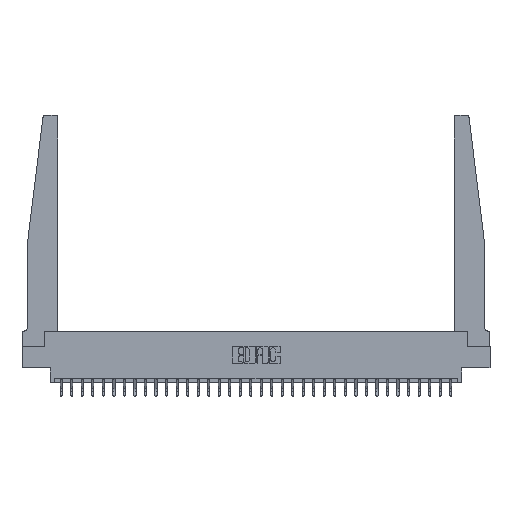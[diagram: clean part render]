
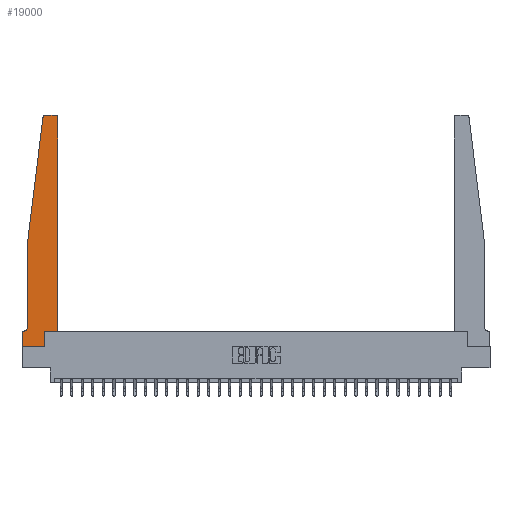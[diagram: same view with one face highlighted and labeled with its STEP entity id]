
A CAD part, top view. The second image highlights one B-rep face of the part: STEP entity #19000.
In plain terms, the highlighted planar face has unit normal (0, 0, 1).
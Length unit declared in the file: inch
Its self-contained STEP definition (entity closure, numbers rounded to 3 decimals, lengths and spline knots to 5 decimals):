
#228 = ORIENTED_EDGE ( 'NONE', *, *, #20052, .T. ) ;
#772 = CARTESIAN_POINT ( 'NONE',  ( 0.2605, 0.18, 0.37 ) ) ;
#920 = DIRECTION ( 'NONE',  ( 0., 1., 0. ) ) ;
#1320 = ORIENTED_EDGE ( 'NONE', *, *, #6253, .T. ) ;
#2026 = VECTOR ( 'NONE', #7015, 39.37008 ) ;
#2104 = AXIS2_PLACEMENT_3D ( 'NONE', #2556, #12099, #26341 ) ;
#2418 = VERTEX_POINT ( 'NONE', #26243 ) ;
#2556 = CARTESIAN_POINT ( 'NONE',  ( 0.015, 0.2375, 0.37 ) ) ;
#3016 = CARTESIAN_POINT ( 'NONE',  ( 0.425, 2.72, 0.37 ) ) ;
#3217 = LINE ( 'NONE', #29176, #16742 ) ;
#3379 = ORIENTED_EDGE ( 'NONE', *, *, #28128, .T. ) ;
#3583 = VERTEX_POINT ( 'NONE', #9162 ) ;
#3828 = DIRECTION ( 'NONE',  ( 1., 0., 0. ) ) ;
#4292 = VECTOR ( 'NONE', #920, 39.37008 ) ;
#4565 = CARTESIAN_POINT ( 'NONE',  ( 0.27653, 2.72, 0.37 ) ) ;
#4827 = EDGE_CURVE ( 'NONE', #3583, #15010, #14990, .T. ) ;
#4882 = DIRECTION ( 'NONE',  ( 1., 0., 0. ) ) ;
#4998 = CIRCLE ( 'NONE', #2104, 0.05 ) ;
#5313 = LINE ( 'NONE', #772, #13185 ) ;
#5626 = CARTESIAN_POINT ( 'NONE',  ( 0.425, 0.18, 0.37 ) ) ;
#5754 = DIRECTION ( 'NONE',  ( 0., 0., 1. ) ) ;
#5775 = CARTESIAN_POINT ( 'NONE',  ( 0.425, 0.18, 0.37 ) ) ;
#6186 = CARTESIAN_POINT ( 'NONE',  ( 0., 0.1875, 0.37 ) ) ;
#6253 = EDGE_CURVE ( 'NONE', #8029, #3583, #12339, .T. ) ;
#7015 = DIRECTION ( 'NONE',  ( 0., -1., 0. ) ) ;
#7041 = EDGE_CURVE ( 'NONE', #10366, #22657, #21961, .T. ) ;
#7259 = CIRCLE ( 'NONE', #21730, 0.03 ) ;
#7841 = CARTESIAN_POINT ( 'NONE',  ( 0.27653, 2.75, 0.37 ) ) ;
#8029 = VERTEX_POINT ( 'NONE', #20749 ) ;
#8044 = VERTEX_POINT ( 'NONE', #16354 ) ;
#8095 = LINE ( 'NONE', #12914, #13352 ) ;
#8832 = VERTEX_POINT ( 'NONE', #19907 ) ;
#9162 = CARTESIAN_POINT ( 'NONE',  ( 0.425, 0.18, 0.37 ) ) ;
#9662 = LINE ( 'NONE', #16986, #2026 ) ;
#9875 = ORIENTED_EDGE ( 'NONE', *, *, #13506, .T. ) ;
#10366 = VERTEX_POINT ( 'NONE', #27850 ) ;
#10538 = ORIENTED_EDGE ( 'NONE', *, *, #28315, .T. ) ;
#10979 = VECTOR ( 'NONE', #12352, 39.37008 ) ;
#11277 = VECTOR ( 'NONE', #29229, 39.37008 ) ;
#11292 = CIRCLE ( 'NONE', #11801, 0.03 ) ;
#11801 = AXIS2_PLACEMENT_3D ( 'NONE', #29205, #5754, #29053 ) ;
#11975 = ORIENTED_EDGE ( 'NONE', *, *, #13963, .T. ) ;
#12059 = VERTEX_POINT ( 'NONE', #25987 ) ;
#12060 = LINE ( 'NONE', #29104, #24418 ) ;
#12099 = DIRECTION ( 'NONE',  ( 0., 0., -1. ) ) ;
#12259 = EDGE_CURVE ( 'NONE', #12869, #8029, #5313, .T. ) ;
#12339 = LINE ( 'NONE', #5626, #11277 ) ;
#12352 = DIRECTION ( 'NONE',  ( -1., 0., 0. ) ) ;
#12611 = DIRECTION ( 'NONE',  ( 0., -1., 0. ) ) ;
#12739 = DIRECTION ( 'NONE',  ( -0.122, -0.992, 0. ) ) ;
#12869 = VERTEX_POINT ( 'NONE', #27484 ) ;
#12914 = CARTESIAN_POINT ( 'NONE',  ( 0.065, 1.25, 0.37 ) ) ;
#13185 = VECTOR ( 'NONE', #24089, 39.37008 ) ;
#13352 = VECTOR ( 'NONE', #12611, 39.37008 ) ;
#13506 = EDGE_CURVE ( 'NONE', #22657, #8832, #7259, .T. ) ;
#13808 = FACE_OUTER_BOUND ( 'NONE', #25601, .T. ) ;
#13877 = CARTESIAN_POINT ( 'NONE',  ( 0.015, 0.1875, 0.37 ) ) ;
#13963 = EDGE_CURVE ( 'NONE', #15010, #10366, #11292, .T. ) ;
#14781 = VECTOR ( 'NONE', #29008, 39.37008 ) ;
#14919 = CARTESIAN_POINT ( 'NONE',  ( 0.25, 2.75, 0.37 ) ) ;
#14990 = LINE ( 'NONE', #5775, #4292 ) ;
#15010 = VERTEX_POINT ( 'NONE', #3016 ) ;
#15713 = DIRECTION ( 'NONE',  ( 0., 0., 1. ) ) ;
#16354 = CARTESIAN_POINT ( 'NONE',  ( 0., 0., 0.37 ) ) ;
#16742 = VECTOR ( 'NONE', #12739, 39.37008 ) ;
#16812 = VERTEX_POINT ( 'NONE', #13877 ) ;
#16986 = CARTESIAN_POINT ( 'NONE',  ( 0., 0., 0.37 ) ) ;
#19000 = ADVANCED_FACE ( 'NONE', ( #13808 ), #27603, .T. ) ;
#19087 = DIRECTION ( 'NONE',  ( 0., 0., 1. ) ) ;
#19552 = VERTEX_POINT ( 'NONE', #25149 ) ;
#19609 = ORIENTED_EDGE ( 'NONE', *, *, #12259, .T. ) ;
#19646 = ORIENTED_EDGE ( 'NONE', *, *, #25704, .T. ) ;
#19907 = CARTESIAN_POINT ( 'NONE',  ( 0.24675, 2.72367, 0.37 ) ) ;
#20052 = EDGE_CURVE ( 'NONE', #8832, #2418, #3217, .T. ) ;
#20749 = CARTESIAN_POINT ( 'NONE',  ( 0.2605, 0.18, 0.37 ) ) ;
#21591 = CARTESIAN_POINT ( 'NONE',  ( 0.065, 0.1875, 0.37 ) ) ;
#21730 = AXIS2_PLACEMENT_3D ( 'NONE', #4565, #19087, #28182 ) ;
#21961 = LINE ( 'NONE', #14919, #14781 ) ;
#22657 = VERTEX_POINT ( 'NONE', #7841 ) ;
#23864 = ORIENTED_EDGE ( 'NONE', *, *, #30018, .T. ) ;
#24089 = DIRECTION ( 'NONE',  ( 0., 1., 0. ) ) ;
#24168 = ORIENTED_EDGE ( 'NONE', *, *, #28801, .T. ) ;
#24418 = VECTOR ( 'NONE', #4882, 39.37008 ) ;
#25149 = CARTESIAN_POINT ( 'NONE',  ( 0.065, 0.2375, 0.37 ) ) ;
#25601 = EDGE_LOOP ( 'NONE', ( #30572, #9875, #228, #19646, #23864, #10538, #3379, #24168, #19609, #1320, #30736, #11975 ) ) ;
#25704 = EDGE_CURVE ( 'NONE', #2418, #19552, #8095, .T. ) ;
#25987 = CARTESIAN_POINT ( 'NONE',  ( 0., 0.1875, 0.37 ) ) ;
#26243 = CARTESIAN_POINT ( 'NONE',  ( 0.065, 1.25, 0.37 ) ) ;
#26341 = DIRECTION ( 'NONE',  ( -1., 0., 0. ) ) ;
#26905 = LINE ( 'NONE', #21591, #10979 ) ;
#27484 = CARTESIAN_POINT ( 'NONE',  ( 0.2605, 0., 0.37 ) ) ;
#27603 = PLANE ( 'NONE',  #27688 ) ;
#27688 = AXIS2_PLACEMENT_3D ( 'NONE', #6186, #15713, #3828 ) ;
#27850 = CARTESIAN_POINT ( 'NONE',  ( 0.395, 2.75, 0.37 ) ) ;
#28128 = EDGE_CURVE ( 'NONE', #12059, #8044, #9662, .T. ) ;
#28182 = DIRECTION ( 'NONE',  ( 1., 0., 0. ) ) ;
#28315 = EDGE_CURVE ( 'NONE', #16812, #12059, #26905, .T. ) ;
#28801 = EDGE_CURVE ( 'NONE', #8044, #12869, #12060, .T. ) ;
#29008 = DIRECTION ( 'NONE',  ( -1., 0., 0. ) ) ;
#29053 = DIRECTION ( 'NONE',  ( 1., 0., 0. ) ) ;
#29104 = CARTESIAN_POINT ( 'NONE',  ( 0., 0., 0.37 ) ) ;
#29176 = CARTESIAN_POINT ( 'NONE',  ( 0.065, 1.25, 0.37 ) ) ;
#29205 = CARTESIAN_POINT ( 'NONE',  ( 0.395, 2.72, 0.37 ) ) ;
#29229 = DIRECTION ( 'NONE',  ( 1., 0., 0. ) ) ;
#30018 = EDGE_CURVE ( 'NONE', #19552, #16812, #4998, .T. ) ;
#30572 = ORIENTED_EDGE ( 'NONE', *, *, #7041, .T. ) ;
#30736 = ORIENTED_EDGE ( 'NONE', *, *, #4827, .T. ) ;
